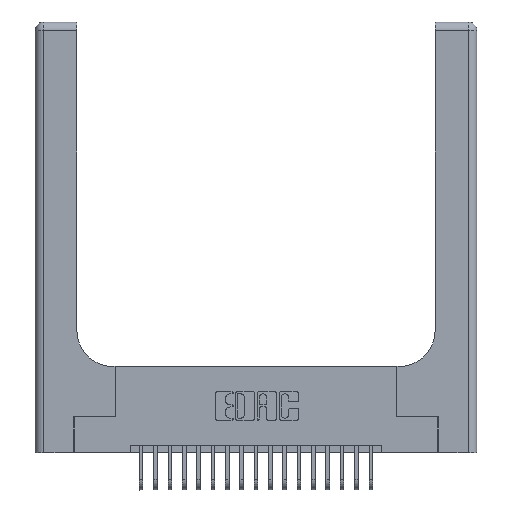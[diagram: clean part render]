
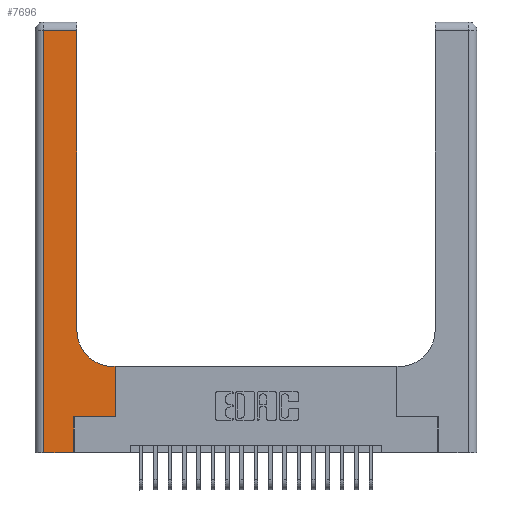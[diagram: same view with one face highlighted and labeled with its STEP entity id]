
A CAD part, top view. The second image highlights one B-rep face of the part: STEP entity #7696.
In plain terms, the highlighted planar face has unit normal (0, 0, 1).
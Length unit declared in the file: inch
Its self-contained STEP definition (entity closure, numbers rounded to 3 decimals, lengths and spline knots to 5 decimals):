
#371 = CARTESIAN_POINT ( 'NONE',  ( 0.06, 2.94, 0.37 ) ) ;
#455 = EDGE_CURVE ( 'NONE', #18400, #20267, #19510, .T. ) ;
#467 = CARTESIAN_POINT ( 'NONE',  ( 0.5585, 0.6, 0.37 ) ) ;
#556 = DIRECTION ( 'NONE',  ( -1., 0., 0. ) ) ;
#650 = ORIENTED_EDGE ( 'NONE', *, *, #18464, .T. ) ;
#1212 = ORIENTED_EDGE ( 'NONE', *, *, #8763, .T. ) ;
#1430 = CARTESIAN_POINT ( 'NONE',  ( 0.269, 0.25, 0.37 ) ) ;
#1455 = CARTESIAN_POINT ( 'NONE',  ( 0.06, 0., 0.37 ) ) ;
#1727 = CARTESIAN_POINT ( 'NONE',  ( 0.2915, 0.85, 0.37 ) ) ;
#1884 = VECTOR ( 'NONE', #20702, 39.37008 ) ;
#2050 = VERTEX_POINT ( 'NONE', #371 ) ;
#3340 = LINE ( 'NONE', #12406, #7243 ) ;
#4262 = DIRECTION ( 'NONE',  ( 0., 1., 0. ) ) ;
#4386 = VERTEX_POINT ( 'NONE', #5337 ) ;
#4797 = DIRECTION ( 'NONE',  ( 0., 1., 0. ) ) ;
#5337 = CARTESIAN_POINT ( 'NONE',  ( 0.2915, 2.94, 0.37 ) ) ;
#5431 = DIRECTION ( 'NONE',  ( 0., 0., -1. ) ) ;
#5478 = VERTEX_POINT ( 'NONE', #6627 ) ;
#5969 = CARTESIAN_POINT ( 'NONE',  ( 0.5415, 0.6, 0.37 ) ) ;
#6253 = ORIENTED_EDGE ( 'NONE', *, *, #455, .T. ) ;
#6344 = LINE ( 'NONE', #19045, #1884 ) ;
#6627 = CARTESIAN_POINT ( 'NONE',  ( 0.5585, 0.25, 0.37 ) ) ;
#6995 = VECTOR ( 'NONE', #11872, 39.37008 ) ;
#7243 = VECTOR ( 'NONE', #10716, 39.37008 ) ;
#7534 = CARTESIAN_POINT ( 'NONE',  ( 0.2915, 3., 0.37 ) ) ;
#7696 = ADVANCED_FACE ( 'NONE', ( #11879 ), #9850, .F. ) ;
#7846 = VERTEX_POINT ( 'NONE', #13824 ) ;
#7885 = CARTESIAN_POINT ( 'NONE',  ( 0.269, 0.25, 0.37 ) ) ;
#8763 = EDGE_CURVE ( 'NONE', #20267, #4386, #16993, .T. ) ;
#9119 = LINE ( 'NONE', #1430, #17373 ) ;
#9376 = ORIENTED_EDGE ( 'NONE', *, *, #10017, .T. ) ;
#9378 = CARTESIAN_POINT ( 'NONE',  ( 0.06, 3., 0.37 ) ) ;
#9447 = DIRECTION ( 'NONE',  ( 0., -1., 0. ) ) ;
#9850 = PLANE ( 'NONE',  #16256 ) ;
#9905 = ORIENTED_EDGE ( 'NONE', *, *, #17494, .T. ) ;
#9929 = DIRECTION ( 'NONE',  ( -1., 0., 0. ) ) ;
#10017 = EDGE_CURVE ( 'NONE', #15264, #7846, #6344, .T. ) ;
#10716 = DIRECTION ( 'NONE',  ( 0., 1., 0. ) ) ;
#10846 = LINE ( 'NONE', #9378, #19099 ) ;
#11162 = VERTEX_POINT ( 'NONE', #467 ) ;
#11473 = VECTOR ( 'NONE', #556, 39.37008 ) ;
#11872 = DIRECTION ( 'NONE',  ( -1., 0., 0. ) ) ;
#11879 = FACE_OUTER_BOUND ( 'NONE', #21090, .T. ) ;
#11918 = LINE ( 'NONE', #16773, #6995 ) ;
#12406 = CARTESIAN_POINT ( 'NONE',  ( 0.269, 0., 0.37 ) ) ;
#12655 = VECTOR ( 'NONE', #4262, 39.37008 ) ;
#13091 = CARTESIAN_POINT ( 'NONE',  ( 0.5585, 0.25, 0.37 ) ) ;
#13824 = CARTESIAN_POINT ( 'NONE',  ( 0.269, 0., 0.37 ) ) ;
#15014 = ORIENTED_EDGE ( 'NONE', *, *, #15270, .T. ) ;
#15264 = VERTEX_POINT ( 'NONE', #1455 ) ;
#15270 = EDGE_CURVE ( 'NONE', #5478, #11162, #18433, .T. ) ;
#15367 = CARTESIAN_POINT ( 'NONE',  ( 0.5415, 0.85, 0.37 ) ) ;
#15773 = EDGE_CURVE ( 'NONE', #17864, #5478, #9119, .T. ) ;
#16094 = EDGE_CURVE ( 'NONE', #4386, #2050, #16375, .T. ) ;
#16256 = AXIS2_PLACEMENT_3D ( 'NONE', #19756, #19831, #9929 ) ;
#16375 = LINE ( 'NONE', #20382, #11473 ) ;
#16773 = CARTESIAN_POINT ( 'NONE',  ( 0.2915, 0.6, 0.37 ) ) ;
#16993 = LINE ( 'NONE', #7534, #12655 ) ;
#17004 = DIRECTION ( 'NONE',  ( 1., 0., 0. ) ) ;
#17280 = ORIENTED_EDGE ( 'NONE', *, *, #15773, .T. ) ;
#17373 = VECTOR ( 'NONE', #21265, 39.37008 ) ;
#17494 = EDGE_CURVE ( 'NONE', #11162, #18400, #11918, .T. ) ;
#17713 = EDGE_CURVE ( 'NONE', #7846, #17864, #3340, .T. ) ;
#17864 = VERTEX_POINT ( 'NONE', #7885 ) ;
#18235 = AXIS2_PLACEMENT_3D ( 'NONE', #15367, #5431, #17004 ) ;
#18400 = VERTEX_POINT ( 'NONE', #5969 ) ;
#18433 = LINE ( 'NONE', #13091, #18959 ) ;
#18464 = EDGE_CURVE ( 'NONE', #2050, #15264, #10846, .T. ) ;
#18959 = VECTOR ( 'NONE', #4797, 39.37008 ) ;
#19015 = ORIENTED_EDGE ( 'NONE', *, *, #16094, .T. ) ;
#19045 = CARTESIAN_POINT ( 'NONE',  ( 0., 0., 0.37 ) ) ;
#19099 = VECTOR ( 'NONE', #9447, 39.37008 ) ;
#19356 = ORIENTED_EDGE ( 'NONE', *, *, #17713, .T. ) ;
#19510 = CIRCLE ( 'NONE', #18235, 0.25 ) ;
#19756 = CARTESIAN_POINT ( 'NONE',  ( 0., 3., 0.37 ) ) ;
#19831 = DIRECTION ( 'NONE',  ( 0., 0., -1. ) ) ;
#20267 = VERTEX_POINT ( 'NONE', #1727 ) ;
#20382 = CARTESIAN_POINT ( 'NONE',  ( 0., 2.94, 0.37 ) ) ;
#20702 = DIRECTION ( 'NONE',  ( 1., 0., 0. ) ) ;
#21090 = EDGE_LOOP ( 'NONE', ( #1212, #19015, #650, #9376, #19356, #17280, #15014, #9905, #6253 ) ) ;
#21265 = DIRECTION ( 'NONE',  ( 1., 0., 0. ) ) ;
